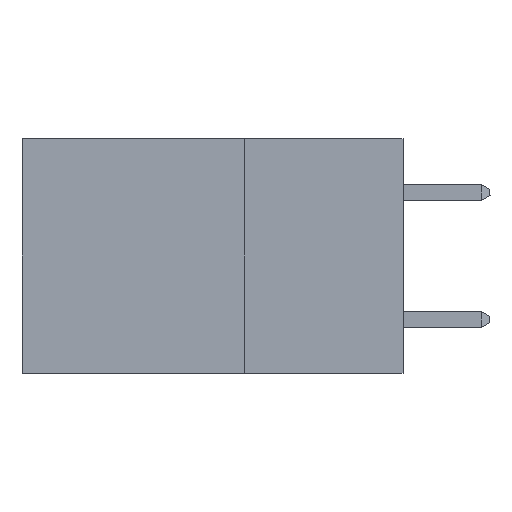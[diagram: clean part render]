
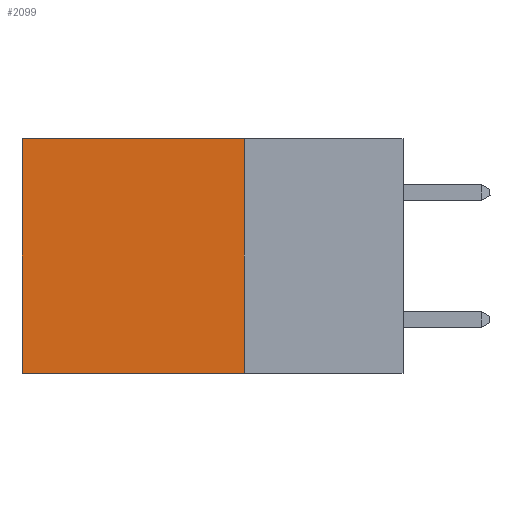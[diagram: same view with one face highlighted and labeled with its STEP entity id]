
A CAD part, left-side view. The second image highlights one B-rep face of the part: STEP entity #2099.
In plain terms, the highlighted planar face has unit normal (-1, 0, 0).
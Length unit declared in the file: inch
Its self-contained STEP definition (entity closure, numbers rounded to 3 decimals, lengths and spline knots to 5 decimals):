
#1123 = CARTESIAN_POINT ( 'NONE',  ( 0.2875, 0.25, -0.37 ) ) ;
#2079 = VECTOR ( 'NONE', #36269, 39.37008 ) ;
#2099 = ADVANCED_FACE ( 'NONE', ( #23441 ), #32817, .F. ) ;
#2568 = CARTESIAN_POINT ( 'NONE',  ( 0.2875, 0.25, 0. ) ) ;
#7287 = LINE ( 'NONE', #11049, #2079 ) ;
#8444 = CARTESIAN_POINT ( 'NONE',  ( 0.2875, 0.25, 0. ) ) ;
#9214 = VERTEX_POINT ( 'NONE', #13319 ) ;
#9519 = VERTEX_POINT ( 'NONE', #19073 ) ;
#10526 = DIRECTION ( 'NONE',  ( 0., 0., -1. ) ) ;
#11049 = CARTESIAN_POINT ( 'NONE',  ( 0.2875, 0.6, 0. ) ) ;
#13153 = VERTEX_POINT ( 'NONE', #36266 ) ;
#13319 = CARTESIAN_POINT ( 'NONE',  ( 0.2875, 0.6, -0.37 ) ) ;
#13367 = EDGE_LOOP ( 'NONE', ( #30165, #24899, #37950, #16592 ) ) ;
#13462 = CARTESIAN_POINT ( 'NONE',  ( 0.2875, 0.25, 0. ) ) ;
#15513 = DIRECTION ( 'NONE',  ( 0., 1., 0. ) ) ;
#16592 = ORIENTED_EDGE ( 'NONE', *, *, #30348, .T. ) ;
#18297 = VECTOR ( 'NONE', #15513, 39.37008 ) ;
#18956 = VECTOR ( 'NONE', #36370, 39.37008 ) ;
#19073 = CARTESIAN_POINT ( 'NONE',  ( 0.2875, 0.25, -0.37 ) ) ;
#19309 = CARTESIAN_POINT ( 'NONE',  ( 0.2875, 0.6, 0. ) ) ;
#21577 = VECTOR ( 'NONE', #24278, 39.37008 ) ;
#22735 = VERTEX_POINT ( 'NONE', #19309 ) ;
#23026 = DIRECTION ( 'NONE',  ( 1., 0., 0. ) ) ;
#23441 = FACE_OUTER_BOUND ( 'NONE', #13367, .T. ) ;
#24278 = DIRECTION ( 'NONE',  ( 0., 0., -1. ) ) ;
#24899 = ORIENTED_EDGE ( 'NONE', *, *, #30100, .F. ) ;
#25030 = EDGE_CURVE ( 'NONE', #22735, #9214, #7287, .T. ) ;
#30100 = EDGE_CURVE ( 'NONE', #9519, #9214, #35957, .T. ) ;
#30165 = ORIENTED_EDGE ( 'NONE', *, *, #25030, .T. ) ;
#30348 = EDGE_CURVE ( 'NONE', #13153, #22735, #40352, .T. ) ;
#32817 = PLANE ( 'NONE',  #40913 ) ;
#32858 = EDGE_CURVE ( 'NONE', #13153, #9519, #33233, .T. ) ;
#33233 = LINE ( 'NONE', #8444, #21577 ) ;
#35957 = LINE ( 'NONE', #1123, #18956 ) ;
#36266 = CARTESIAN_POINT ( 'NONE',  ( 0.2875, 0.25, 0. ) ) ;
#36269 = DIRECTION ( 'NONE',  ( 0., 0., -1. ) ) ;
#36370 = DIRECTION ( 'NONE',  ( 0., 1., 0. ) ) ;
#37950 = ORIENTED_EDGE ( 'NONE', *, *, #32858, .F. ) ;
#40352 = LINE ( 'NONE', #2568, #18297 ) ;
#40913 = AXIS2_PLACEMENT_3D ( 'NONE', #13462, #23026, #10526 ) ;
